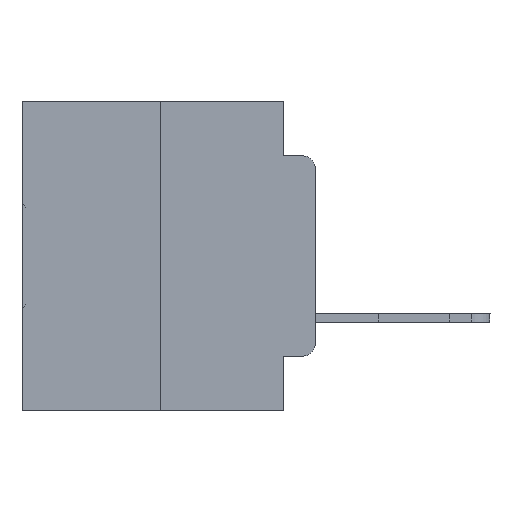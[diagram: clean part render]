
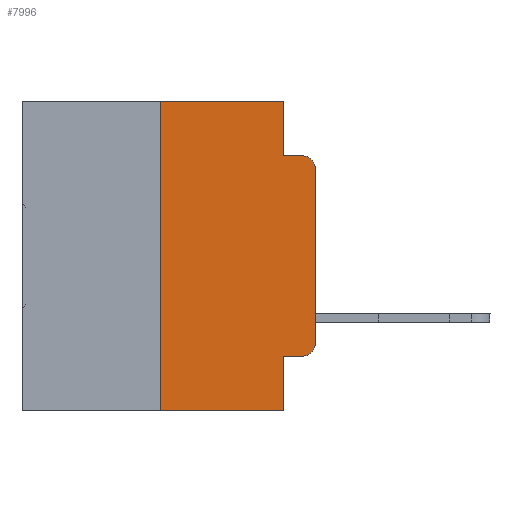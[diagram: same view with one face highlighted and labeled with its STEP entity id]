
A CAD part, left-side view. The second image highlights one B-rep face of the part: STEP entity #7996.
In plain terms, the highlighted planar face has unit normal (-1, 0, 0).
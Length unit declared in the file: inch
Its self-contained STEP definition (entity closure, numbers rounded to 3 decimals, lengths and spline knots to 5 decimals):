
#1593 = CARTESIAN_POINT ( 'NONE',  ( 0., 0., -0.1085 ) ) ;
#1814 = VECTOR ( 'NONE', #13051, 39.37008 ) ;
#2738 = PLANE ( 'NONE',  #21067 ) ;
#2932 = CARTESIAN_POINT ( 'NONE',  ( 0., 0.473, 0. ) ) ;
#3533 = DIRECTION ( 'NONE',  ( -1., 0., 0. ) ) ;
#3639 = CARTESIAN_POINT ( 'NONE',  ( 0., 0.02, -0.3915 ) ) ;
#3685 = VERTEX_POINT ( 'NONE', #22350 ) ;
#5282 = FACE_OUTER_BOUND ( 'NONE', #23939, .T. ) ;
#5347 = VERTEX_POINT ( 'NONE', #18375 ) ;
#5534 = VECTOR ( 'NONE', #11452, 39.37008 ) ;
#5686 = VERTEX_POINT ( 'NONE', #7273 ) ;
#5736 = VECTOR ( 'NONE', #10856, 39.37008 ) ;
#6024 = CARTESIAN_POINT ( 'NONE',  ( 0., 0.051, 0. ) ) ;
#7273 = CARTESIAN_POINT ( 'NONE',  ( 0., 0.051, 0. ) ) ;
#7996 = ADVANCED_FACE ( 'NONE', ( #5282 ), #2738, .F. ) ;
#8247 = CARTESIAN_POINT ( 'NONE',  ( 0., 0.051, -0.0885 ) ) ;
#8405 = CARTESIAN_POINT ( 'NONE',  ( 0., 0.051, 0. ) ) ;
#8616 = EDGE_CURVE ( 'NONE', #28754, #20198, #17036, .T. ) ;
#9201 = LINE ( 'NONE', #8405, #5736 ) ;
#9488 = CARTESIAN_POINT ( 'NONE',  ( 0., 0.051, -0.0885 ) ) ;
#9772 = AXIS2_PLACEMENT_3D ( 'NONE', #3639, #3533, #30346 ) ;
#9986 = DIRECTION ( 'NONE',  ( 0., 0., -1. ) ) ;
#10856 = DIRECTION ( 'NONE',  ( 0., 0., -1. ) ) ;
#11452 = DIRECTION ( 'NONE',  ( 0., 0., 1. ) ) ;
#11555 = ORIENTED_EDGE ( 'NONE', *, *, #13319, .F. ) ;
#11688 = ORIENTED_EDGE ( 'NONE', *, *, #8616, .F. ) ;
#12084 = CARTESIAN_POINT ( 'NONE',  ( 0., 0.25, -0.5 ) ) ;
#12269 = EDGE_CURVE ( 'NONE', #18012, #24312, #9201, .T. ) ;
#13051 = DIRECTION ( 'NONE',  ( 0., -1., 0. ) ) ;
#13280 = EDGE_CURVE ( 'NONE', #18012, #3685, #29153, .T. ) ;
#13319 = EDGE_CURVE ( 'NONE', #15044, #24036, #15417, .T. ) ;
#13390 = ORIENTED_EDGE ( 'NONE', *, *, #26948, .F. ) ;
#13575 = CIRCLE ( 'NONE', #9772, 0.02 ) ;
#14345 = VECTOR ( 'NONE', #25352, 39.37008 ) ;
#15044 = VERTEX_POINT ( 'NONE', #12084 ) ;
#15236 = VECTOR ( 'NONE', #19114, 39.37008 ) ;
#15243 = AXIS2_PLACEMENT_3D ( 'NONE', #29687, #25922, #15902 ) ;
#15347 = CARTESIAN_POINT ( 'NONE',  ( 0., 0.051, -0.4115 ) ) ;
#15417 = LINE ( 'NONE', #18006, #5534 ) ;
#15902 = DIRECTION ( 'NONE',  ( 0., 0., -1. ) ) ;
#16043 = EDGE_CURVE ( 'NONE', #5347, #18511, #23229, .T. ) ;
#16386 = VECTOR ( 'NONE', #30294, 39.37008 ) ;
#16453 = CARTESIAN_POINT ( 'NONE',  ( 0., 0., 0. ) ) ;
#16647 = CARTESIAN_POINT ( 'NONE',  ( 0., 0.25, 0. ) ) ;
#17036 = LINE ( 'NONE', #8247, #1814 ) ;
#17089 = DIRECTION ( 'NONE',  ( 0., -1., 0. ) ) ;
#17186 = CARTESIAN_POINT ( 'NONE',  ( 0., 0.473, 0. ) ) ;
#18006 = CARTESIAN_POINT ( 'NONE',  ( 0., 0.25, 0. ) ) ;
#18012 = VERTEX_POINT ( 'NONE', #28168 ) ;
#18150 = LINE ( 'NONE', #6024, #19677 ) ;
#18154 = CARTESIAN_POINT ( 'NONE',  ( 0., 0.473, -0.5 ) ) ;
#18375 = CARTESIAN_POINT ( 'NONE',  ( 0., 0., -0.3915 ) ) ;
#18511 = VERTEX_POINT ( 'NONE', #1593 ) ;
#18841 = ORIENTED_EDGE ( 'NONE', *, *, #13280, .T. ) ;
#19114 = DIRECTION ( 'NONE',  ( 0., 0., 1. ) ) ;
#19677 = VECTOR ( 'NONE', #23123, 39.37008 ) ;
#19737 = ORIENTED_EDGE ( 'NONE', *, *, #12269, .F. ) ;
#19956 = DIRECTION ( 'NONE',  ( 1., 0., 0. ) ) ;
#20052 = ORIENTED_EDGE ( 'NONE', *, *, #23816, .F. ) ;
#20198 = VERTEX_POINT ( 'NONE', #25365 ) ;
#20225 = LINE ( 'NONE', #17186, #26340 ) ;
#21067 = AXIS2_PLACEMENT_3D ( 'NONE', #2932, #19956, #9986 ) ;
#21923 = EDGE_CURVE ( 'NONE', #15044, #24312, #26291, .T. ) ;
#21949 = ORIENTED_EDGE ( 'NONE', *, *, #24638, .T. ) ;
#22267 = CIRCLE ( 'NONE', #15243, 0.02 ) ;
#22350 = CARTESIAN_POINT ( 'NONE',  ( 0., 0.02, -0.4115 ) ) ;
#23123 = DIRECTION ( 'NONE',  ( 0., 0., -1. ) ) ;
#23229 = LINE ( 'NONE', #16453, #15236 ) ;
#23816 = EDGE_CURVE ( 'NONE', #5686, #28754, #18150, .T. ) ;
#23939 = EDGE_LOOP ( 'NONE', ( #24796, #21949, #11688, #20052, #13390, #11555, #30973, #19737, #18841, #31527 ) ) ;
#24036 = VERTEX_POINT ( 'NONE', #16647 ) ;
#24312 = VERTEX_POINT ( 'NONE', #29415 ) ;
#24322 = EDGE_CURVE ( 'NONE', #3685, #5347, #13575, .T. ) ;
#24638 = EDGE_CURVE ( 'NONE', #18511, #20198, #22267, .T. ) ;
#24796 = ORIENTED_EDGE ( 'NONE', *, *, #16043, .T. ) ;
#25352 = DIRECTION ( 'NONE',  ( 0., -1., 0. ) ) ;
#25365 = CARTESIAN_POINT ( 'NONE',  ( 0., 0.02, -0.0885 ) ) ;
#25922 = DIRECTION ( 'NONE',  ( -1., 0., 0. ) ) ;
#26291 = LINE ( 'NONE', #18154, #16386 ) ;
#26340 = VECTOR ( 'NONE', #17089, 39.37008 ) ;
#26948 = EDGE_CURVE ( 'NONE', #24036, #5686, #20225, .T. ) ;
#28168 = CARTESIAN_POINT ( 'NONE',  ( 0., 0.051, -0.4115 ) ) ;
#28754 = VERTEX_POINT ( 'NONE', #9488 ) ;
#29153 = LINE ( 'NONE', #15347, #14345 ) ;
#29415 = CARTESIAN_POINT ( 'NONE',  ( 0., 0.051, -0.5 ) ) ;
#29687 = CARTESIAN_POINT ( 'NONE',  ( 0., 0.02, -0.1085 ) ) ;
#30294 = DIRECTION ( 'NONE',  ( 0., -1., 0. ) ) ;
#30346 = DIRECTION ( 'NONE',  ( 0., 0., -1. ) ) ;
#30973 = ORIENTED_EDGE ( 'NONE', *, *, #21923, .T. ) ;
#31527 = ORIENTED_EDGE ( 'NONE', *, *, #24322, .T. ) ;
